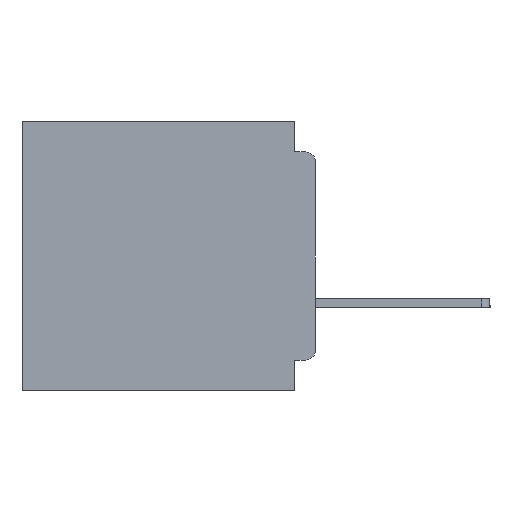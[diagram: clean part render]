
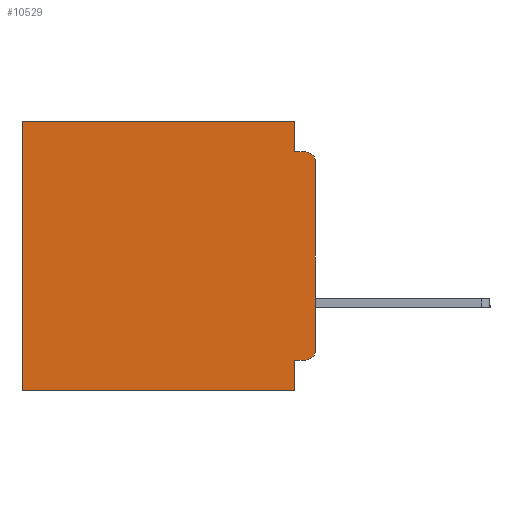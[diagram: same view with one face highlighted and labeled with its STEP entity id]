
A CAD part, left-side view. The second image highlights one B-rep face of the part: STEP entity #10529.
In plain terms, the highlighted planar face has unit normal (-1, 0, 0).
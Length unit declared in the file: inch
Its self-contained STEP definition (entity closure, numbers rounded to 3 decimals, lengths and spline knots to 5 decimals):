
#4 = VERTEX_POINT ( 'NONE', #40246 ) ;
#861 = LINE ( 'NONE', #52847, #25002 ) ;
#2256 = ORIENTED_EDGE ( 'NONE', *, *, #60976, .F. ) ;
#3417 = EDGE_CURVE ( 'NONE', #31392, #36097, #57367, .T. ) ;
#3920 = CARTESIAN_POINT ( 'NONE',  ( 0.3, 0.437, -0.4 ) ) ;
#3965 = DIRECTION ( 'NONE',  ( 0., 1., 0. ) ) ;
#5729 = PLANE ( 'NONE',  #39876 ) ;
#5976 = DIRECTION ( 'NONE',  ( 0., 0., -1. ) ) ;
#6387 = EDGE_CURVE ( 'NONE', #50419, #36097, #36995, .T. ) ;
#7258 = VECTOR ( 'NONE', #5976, 39.37008 ) ;
#10529 = ADVANCED_FACE ( 'NONE', ( #18554 ), #5729, .F. ) ;
#10579 = DIRECTION ( 'NONE',  ( 0., 0., -1. ) ) ;
#11327 = VERTEX_POINT ( 'NONE', #29737 ) ;
#12015 = CARTESIAN_POINT ( 'NONE',  ( 0.3, 0.015, -0.06 ) ) ;
#12794 = DIRECTION ( 'NONE',  ( 0., 0., -1. ) ) ;
#15131 = EDGE_CURVE ( 'NONE', #50810, #31392, #17421, .T. ) ;
#15625 = CARTESIAN_POINT ( 'NONE',  ( 0.3, 0.015, -0.34 ) ) ;
#16024 = VECTOR ( 'NONE', #45721, 39.37008 ) ;
#16293 = AXIS2_PLACEMENT_3D ( 'NONE', #15625, #48975, #20469 ) ;
#16860 = DIRECTION ( 'NONE',  ( 0., 0., -1. ) ) ;
#17340 = AXIS2_PLACEMENT_3D ( 'NONE', #12015, #45423, #16860 ) ;
#17361 = CARTESIAN_POINT ( 'NONE',  ( 0.3, 0.031, -0.045 ) ) ;
#17421 = LINE ( 'NONE', #57379, #53827 ) ;
#18554 = FACE_OUTER_BOUND ( 'NONE', #36352, .T. ) ;
#19031 = CARTESIAN_POINT ( 'NONE',  ( 0.3, 0.015, -0.355 ) ) ;
#19524 = EDGE_CURVE ( 'NONE', #11327, #29168, #58212, .T. ) ;
#19592 = CARTESIAN_POINT ( 'NONE',  ( 0.3, 0.437, -0.4 ) ) ;
#20145 = CARTESIAN_POINT ( 'NONE',  ( 0.3, 0., -0.045 ) ) ;
#20469 = DIRECTION ( 'NONE',  ( 0., 0., -1. ) ) ;
#20498 = CIRCLE ( 'NONE', #16293, 0.015 ) ;
#21631 = ORIENTED_EDGE ( 'NONE', *, *, #54952, .T. ) ;
#21958 = ORIENTED_EDGE ( 'NONE', *, *, #15131, .F. ) ;
#24901 = CARTESIAN_POINT ( 'NONE',  ( 0.3, 0., -0.4 ) ) ;
#25002 = VECTOR ( 'NONE', #57547, 39.37008 ) ;
#27097 = CARTESIAN_POINT ( 'NONE',  ( 0.3, 0.031, 0. ) ) ;
#28178 = ORIENTED_EDGE ( 'NONE', *, *, #6387, .T. ) ;
#29168 = VERTEX_POINT ( 'NONE', #3920 ) ;
#29427 = EDGE_CURVE ( 'NONE', #4, #11327, #57858, .T. ) ;
#29598 = DIRECTION ( 'NONE',  ( 0., -1., 0. ) ) ;
#29737 = CARTESIAN_POINT ( 'NONE',  ( 0.3, 0.031, -0.4 ) ) ;
#29962 = CARTESIAN_POINT ( 'NONE',  ( 0.3, 0.031, -0.4 ) ) ;
#30118 = ORIENTED_EDGE ( 'NONE', *, *, #31787, .T. ) ;
#30311 = LINE ( 'NONE', #40975, #16024 ) ;
#31392 = VERTEX_POINT ( 'NONE', #17361 ) ;
#31787 = EDGE_CURVE ( 'NONE', #39069, #43386, #20498, .T. ) ;
#33003 = CARTESIAN_POINT ( 'NONE',  ( 0.3, 0.015, -0.045 ) ) ;
#34031 = VERTEX_POINT ( 'NONE', #41919 ) ;
#35010 = LINE ( 'NONE', #19592, #58582 ) ;
#36097 = VERTEX_POINT ( 'NONE', #33003 ) ;
#36352 = EDGE_LOOP ( 'NONE', ( #58293, #28178, #46639, #21958, #21631, #59344, #52468, #52596, #2256, #30118 ) ) ;
#36995 = CIRCLE ( 'NONE', #17340, 0.015 ) ;
#37516 = CARTESIAN_POINT ( 'NONE',  ( 0.3, 0., -0.4 ) ) ;
#39069 = VERTEX_POINT ( 'NONE', #19031 ) ;
#39283 = DIRECTION ( 'NONE',  ( 1., 0., 0. ) ) ;
#39516 = LINE ( 'NONE', #45999, #60078 ) ;
#39876 = AXIS2_PLACEMENT_3D ( 'NONE', #24901, #39283, #10579 ) ;
#40246 = CARTESIAN_POINT ( 'NONE',  ( 0.3, 0.031, -0.355 ) ) ;
#40975 = CARTESIAN_POINT ( 'NONE',  ( 0.3, 0., -0.355 ) ) ;
#41919 = CARTESIAN_POINT ( 'NONE',  ( 0.3, 0.437, 0. ) ) ;
#43063 = DIRECTION ( 'NONE',  ( 0., 0., -1. ) ) ;
#43386 = VERTEX_POINT ( 'NONE', #44006 ) ;
#44006 = CARTESIAN_POINT ( 'NONE',  ( 0.3, 0., -0.34 ) ) ;
#44924 = VECTOR ( 'NONE', #29598, 39.37008 ) ;
#45423 = DIRECTION ( 'NONE',  ( -1., 0., 0. ) ) ;
#45721 = DIRECTION ( 'NONE',  ( 0., 1., 0. ) ) ;
#45758 = VECTOR ( 'NONE', #3965, 39.37008 ) ;
#45920 = EDGE_CURVE ( 'NONE', #50419, #43386, #39516, .T. ) ;
#45999 = CARTESIAN_POINT ( 'NONE',  ( 0.3, 0., -0.4 ) ) ;
#46639 = ORIENTED_EDGE ( 'NONE', *, *, #3417, .F. ) ;
#48119 = DIRECTION ( 'NONE',  ( 0., 0., -1. ) ) ;
#48975 = DIRECTION ( 'NONE',  ( -1., 0., 0. ) ) ;
#50419 = VERTEX_POINT ( 'NONE', #52574 ) ;
#50810 = VERTEX_POINT ( 'NONE', #27097 ) ;
#52468 = ORIENTED_EDGE ( 'NONE', *, *, #19524, .F. ) ;
#52574 = CARTESIAN_POINT ( 'NONE',  ( 0.3, 0., -0.06 ) ) ;
#52596 = ORIENTED_EDGE ( 'NONE', *, *, #29427, .F. ) ;
#52847 = CARTESIAN_POINT ( 'NONE',  ( 0.3, 0., 0. ) ) ;
#53827 = VECTOR ( 'NONE', #43063, 39.37008 ) ;
#54952 = EDGE_CURVE ( 'NONE', #50810, #34031, #861, .T. ) ;
#57367 = LINE ( 'NONE', #20145, #44924 ) ;
#57379 = CARTESIAN_POINT ( 'NONE',  ( 0.3, 0.031, 0. ) ) ;
#57547 = DIRECTION ( 'NONE',  ( 0., 1., 0. ) ) ;
#57858 = LINE ( 'NONE', #29962, #7258 ) ;
#58212 = LINE ( 'NONE', #37516, #45758 ) ;
#58293 = ORIENTED_EDGE ( 'NONE', *, *, #45920, .F. ) ;
#58582 = VECTOR ( 'NONE', #48119, 39.37008 ) ;
#59190 = EDGE_CURVE ( 'NONE', #34031, #29168, #35010, .T. ) ;
#59344 = ORIENTED_EDGE ( 'NONE', *, *, #59190, .T. ) ;
#60078 = VECTOR ( 'NONE', #12794, 39.37008 ) ;
#60976 = EDGE_CURVE ( 'NONE', #39069, #4, #30311, .T. ) ;
